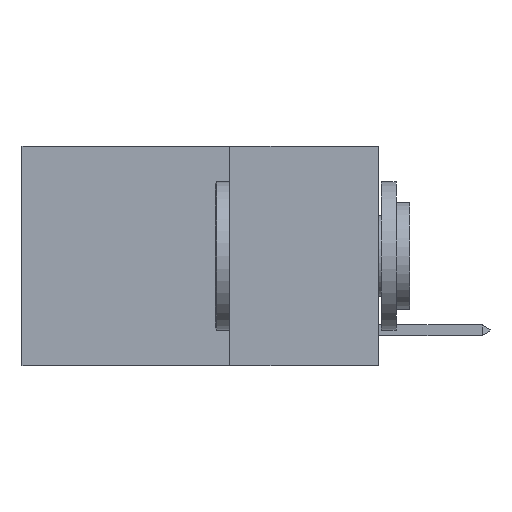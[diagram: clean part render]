
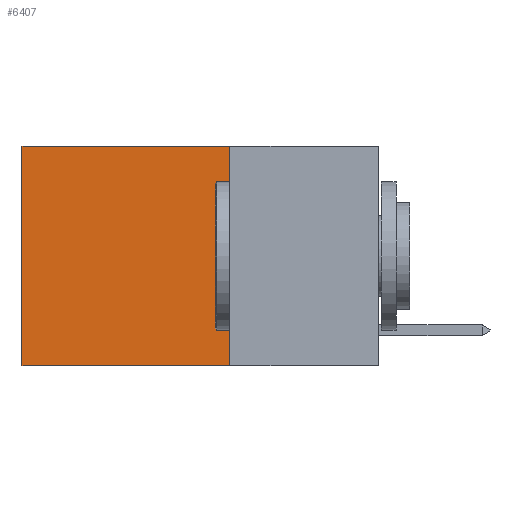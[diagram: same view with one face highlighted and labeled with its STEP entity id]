
A CAD part, left-side view. The second image highlights one B-rep face of the part: STEP entity #6407.
In plain terms, the highlighted planar face has unit normal (-1, 0, 0).
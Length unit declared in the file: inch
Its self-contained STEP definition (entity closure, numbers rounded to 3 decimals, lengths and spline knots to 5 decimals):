
#36 = DIRECTION ( 'NONE',  ( 0., 0., -1. ) ) ;
#571 = CARTESIAN_POINT ( 'NONE',  ( 0.2625, 0.25, 0. ) ) ;
#653 = DIRECTION ( 'NONE',  ( 0., 0., -1. ) ) ;
#821 = LINE ( 'NONE', #9636, #6138 ) ;
#869 = CARTESIAN_POINT ( 'NONE',  ( 0.2625, 0.6, 0. ) ) ;
#1053 = DIRECTION ( 'NONE',  ( 1., 0., 0. ) ) ;
#1133 = VERTEX_POINT ( 'NONE', #9319 ) ;
#1212 = CARTESIAN_POINT ( 'NONE',  ( 0.2625, 0.6, -0.37 ) ) ;
#2091 = VERTEX_POINT ( 'NONE', #869 ) ;
#3291 = ORIENTED_EDGE ( 'NONE', *, *, #3370, .T. ) ;
#3324 = VERTEX_POINT ( 'NONE', #1212 ) ;
#3370 = EDGE_CURVE ( 'NONE', #10929, #2091, #7589, .T. ) ;
#3815 = DIRECTION ( 'NONE',  ( 0., 0., -1. ) ) ;
#4198 = AXIS2_PLACEMENT_3D ( 'NONE', #8833, #1053, #3815 ) ;
#4932 = DIRECTION ( 'NONE',  ( 0., 1., 0. ) ) ;
#5085 = VECTOR ( 'NONE', #653, 39.37008 ) ;
#5180 = VECTOR ( 'NONE', #5931, 39.37008 ) ;
#5372 = PLANE ( 'NONE',  #4198 ) ;
#5931 = DIRECTION ( 'NONE',  ( 0., 1., 0. ) ) ;
#6113 = EDGE_CURVE ( 'NONE', #1133, #3324, #6563, .T. ) ;
#6138 = VECTOR ( 'NONE', #36, 39.37008 ) ;
#6214 = FACE_OUTER_BOUND ( 'NONE', #9182, .T. ) ;
#6407 = ADVANCED_FACE ( 'NONE', ( #6214 ), #5372, .F. ) ;
#6528 = CARTESIAN_POINT ( 'NONE',  ( 0.2625, 0.6, 0. ) ) ;
#6563 = LINE ( 'NONE', #10109, #7025 ) ;
#7025 = VECTOR ( 'NONE', #4932, 39.37008 ) ;
#7299 = ORIENTED_EDGE ( 'NONE', *, *, #10248, .F. ) ;
#7513 = LINE ( 'NONE', #6528, #5085 ) ;
#7589 = LINE ( 'NONE', #8552, #5180 ) ;
#8552 = CARTESIAN_POINT ( 'NONE',  ( 0.2625, 0.25, 0. ) ) ;
#8833 = CARTESIAN_POINT ( 'NONE',  ( 0.2625, 0.25, 0. ) ) ;
#9182 = EDGE_LOOP ( 'NONE', ( #9424, #10440, #7299, #3291 ) ) ;
#9319 = CARTESIAN_POINT ( 'NONE',  ( 0.2625, 0.25, -0.37 ) ) ;
#9424 = ORIENTED_EDGE ( 'NONE', *, *, #10467, .T. ) ;
#9636 = CARTESIAN_POINT ( 'NONE',  ( 0.2625, 0.25, 0. ) ) ;
#10109 = CARTESIAN_POINT ( 'NONE',  ( 0.2625, 0.25, -0.37 ) ) ;
#10248 = EDGE_CURVE ( 'NONE', #10929, #1133, #821, .T. ) ;
#10440 = ORIENTED_EDGE ( 'NONE', *, *, #6113, .F. ) ;
#10467 = EDGE_CURVE ( 'NONE', #2091, #3324, #7513, .T. ) ;
#10929 = VERTEX_POINT ( 'NONE', #571 ) ;
